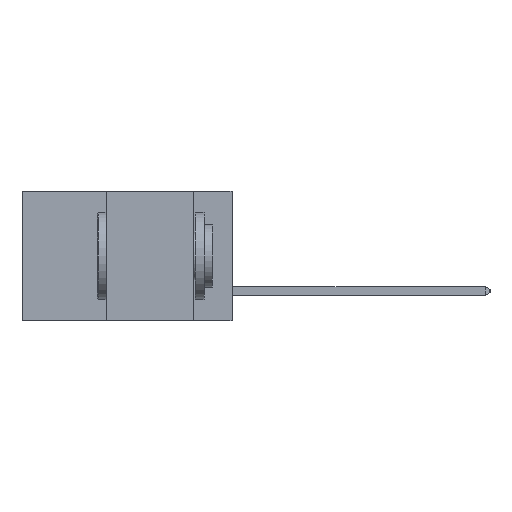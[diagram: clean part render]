
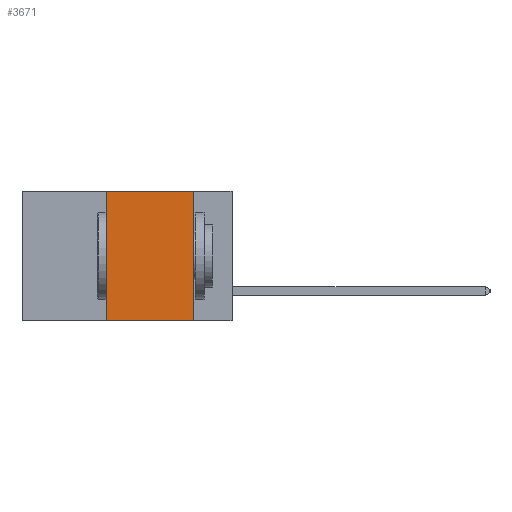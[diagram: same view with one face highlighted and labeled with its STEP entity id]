
A CAD part, left-side view. The second image highlights one B-rep face of the part: STEP entity #3671.
In plain terms, the highlighted planar face has unit normal (-1, 0, 0).
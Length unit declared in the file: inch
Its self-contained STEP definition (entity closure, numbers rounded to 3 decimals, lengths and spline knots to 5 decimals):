
#55 = CARTESIAN_POINT ( 'NONE',  ( 0., 0.6, -0.37 ) ) ;
#513 = DIRECTION ( 'NONE',  ( 0., 0., -1. ) ) ;
#1216 = VECTOR ( 'NONE', #10893, 39.37008 ) ;
#1412 = VERTEX_POINT ( 'NONE', #11977 ) ;
#1413 = DIRECTION ( 'NONE',  ( 0., 0., 1. ) ) ;
#1475 = LINE ( 'NONE', #55, #10325 ) ;
#1529 = CARTESIAN_POINT ( 'NONE',  ( 0., 0.36, 0. ) ) ;
#1856 = ORIENTED_EDGE ( 'NONE', *, *, #12782, .F. ) ;
#2795 = CARTESIAN_POINT ( 'NONE',  ( 0., 0.11, 0. ) ) ;
#3671 = ADVANCED_FACE ( 'NONE', ( #4656 ), #4385, .F. ) ;
#3902 = LINE ( 'NONE', #14279, #1216 ) ;
#4183 = VERTEX_POINT ( 'NONE', #7778 ) ;
#4385 = PLANE ( 'NONE',  #14046 ) ;
#4656 = FACE_OUTER_BOUND ( 'NONE', #12833, .T. ) ;
#4663 = EDGE_CURVE ( 'NONE', #4183, #1412, #9680, .T. ) ;
#6626 = ORIENTED_EDGE ( 'NONE', *, *, #4663, .F. ) ;
#6944 = DIRECTION ( 'NONE',  ( 1., 0., 0. ) ) ;
#6992 = VECTOR ( 'NONE', #1413, 39.37008 ) ;
#7778 = CARTESIAN_POINT ( 'NONE',  ( 0., 0.11, 0. ) ) ;
#8174 = DIRECTION ( 'NONE',  ( 0., -1., 0. ) ) ;
#8444 = EDGE_CURVE ( 'NONE', #11102, #9825, #10030, .T. ) ;
#8830 = ORIENTED_EDGE ( 'NONE', *, *, #8444, .F. ) ;
#8960 = VECTOR ( 'NONE', #513, 39.37008 ) ;
#9680 = LINE ( 'NONE', #2795, #8960 ) ;
#9825 = VERTEX_POINT ( 'NONE', #1529 ) ;
#10030 = LINE ( 'NONE', #12847, #6992 ) ;
#10325 = VECTOR ( 'NONE', #8174, 39.37008 ) ;
#10833 = EDGE_CURVE ( 'NONE', #11102, #1412, #1475, .T. ) ;
#10893 = DIRECTION ( 'NONE',  ( 0., -1., 0. ) ) ;
#11056 = CARTESIAN_POINT ( 'NONE',  ( 0., 0.36, -0.37 ) ) ;
#11102 = VERTEX_POINT ( 'NONE', #11056 ) ;
#11977 = CARTESIAN_POINT ( 'NONE',  ( 0., 0.11, -0.37 ) ) ;
#12398 = CARTESIAN_POINT ( 'NONE',  ( 0., 0.6, 0. ) ) ;
#12782 = EDGE_CURVE ( 'NONE', #9825, #4183, #3902, .T. ) ;
#12833 = EDGE_LOOP ( 'NONE', ( #6626, #1856, #8830, #14075 ) ) ;
#12847 = CARTESIAN_POINT ( 'NONE',  ( 0., 0.36, 0. ) ) ;
#14046 = AXIS2_PLACEMENT_3D ( 'NONE', #12398, #6944, #14911 ) ;
#14075 = ORIENTED_EDGE ( 'NONE', *, *, #10833, .T. ) ;
#14279 = CARTESIAN_POINT ( 'NONE',  ( 0., 0.6, 0. ) ) ;
#14911 = DIRECTION ( 'NONE',  ( 0., 0., -1. ) ) ;
